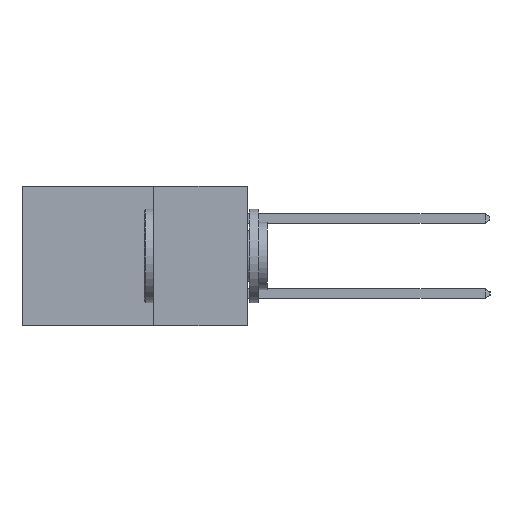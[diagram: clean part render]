
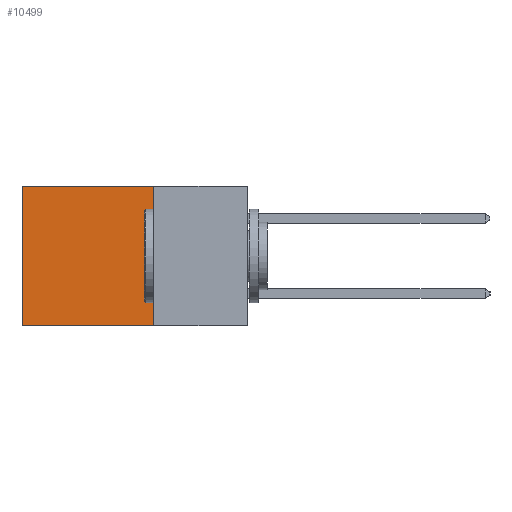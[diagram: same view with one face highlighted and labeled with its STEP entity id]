
A CAD part, left-side view. The second image highlights one B-rep face of the part: STEP entity #10499.
In plain terms, the highlighted planar face has unit normal (-1, 0, 0).
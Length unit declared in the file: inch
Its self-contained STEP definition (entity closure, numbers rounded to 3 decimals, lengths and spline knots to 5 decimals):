
#503 = CARTESIAN_POINT ( 'NONE',  ( 0.2615, 0.6, -0.37 ) ) ;
#1023 = LINE ( 'NONE', #8937, #7380 ) ;
#1083 = DIRECTION ( 'NONE',  ( 1., 0., 0. ) ) ;
#1470 = DIRECTION ( 'NONE',  ( 0., 1., 0. ) ) ;
#1571 = CARTESIAN_POINT ( 'NONE',  ( 0.2615, 0.25, -0.37 ) ) ;
#1933 = ORIENTED_EDGE ( 'NONE', *, *, #5607, .T. ) ;
#2001 = EDGE_CURVE ( 'NONE', #2671, #4017, #1023, .T. ) ;
#2422 = DIRECTION ( 'NONE',  ( 0., 0., -1. ) ) ;
#2440 = DIRECTION ( 'NONE',  ( 0., 1., 0. ) ) ;
#2671 = VERTEX_POINT ( 'NONE', #6411 ) ;
#2825 = VECTOR ( 'NONE', #2422, 39.37008 ) ;
#3660 = DIRECTION ( 'NONE',  ( 0., 0., -1. ) ) ;
#3775 = VECTOR ( 'NONE', #2440, 39.37008 ) ;
#4017 = VERTEX_POINT ( 'NONE', #503 ) ;
#4784 = ORIENTED_EDGE ( 'NONE', *, *, #9238, .F. ) ;
#5200 = CARTESIAN_POINT ( 'NONE',  ( 0.2615, 0.25, -0.37 ) ) ;
#5607 = EDGE_CURVE ( 'NONE', #8441, #6341, #6169, .T. ) ;
#5836 = LINE ( 'NONE', #1571, #2825 ) ;
#5988 = CARTESIAN_POINT ( 'NONE',  ( 0.2615, 0.6, -0.37 ) ) ;
#6169 = LINE ( 'NONE', #6523, #3775 ) ;
#6236 = ORIENTED_EDGE ( 'NONE', *, *, #2001, .F. ) ;
#6341 = VERTEX_POINT ( 'NONE', #10432 ) ;
#6411 = CARTESIAN_POINT ( 'NONE',  ( 0.2615, 0.25, -0.37 ) ) ;
#6523 = CARTESIAN_POINT ( 'NONE',  ( 0.2615, 0.25, 0. ) ) ;
#7016 = VECTOR ( 'NONE', #10147, 39.37008 ) ;
#7242 = EDGE_CURVE ( 'NONE', #6341, #4017, #9463, .T. ) ;
#7380 = VECTOR ( 'NONE', #1470, 39.37008 ) ;
#8000 = ORIENTED_EDGE ( 'NONE', *, *, #7242, .T. ) ;
#8017 = FACE_OUTER_BOUND ( 'NONE', #8414, .T. ) ;
#8414 = EDGE_LOOP ( 'NONE', ( #8000, #6236, #4784, #1933 ) ) ;
#8441 = VERTEX_POINT ( 'NONE', #9095 ) ;
#8937 = CARTESIAN_POINT ( 'NONE',  ( 0.2615, 0.25, -0.37 ) ) ;
#9095 = CARTESIAN_POINT ( 'NONE',  ( 0.2615, 0.25, 0. ) ) ;
#9238 = EDGE_CURVE ( 'NONE', #8441, #2671, #5836, .T. ) ;
#9463 = LINE ( 'NONE', #5988, #7016 ) ;
#10147 = DIRECTION ( 'NONE',  ( 0., 0., -1. ) ) ;
#10192 = PLANE ( 'NONE',  #10313 ) ;
#10313 = AXIS2_PLACEMENT_3D ( 'NONE', #5200, #1083, #3660 ) ;
#10432 = CARTESIAN_POINT ( 'NONE',  ( 0.2615, 0.6, 0. ) ) ;
#10499 = ADVANCED_FACE ( 'NONE', ( #8017 ), #10192, .F. ) ;
